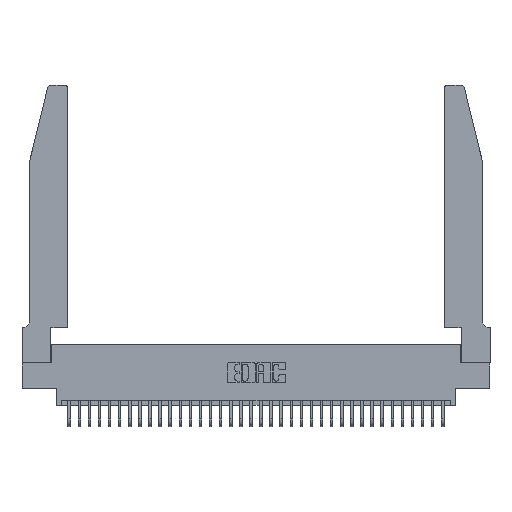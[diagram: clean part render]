
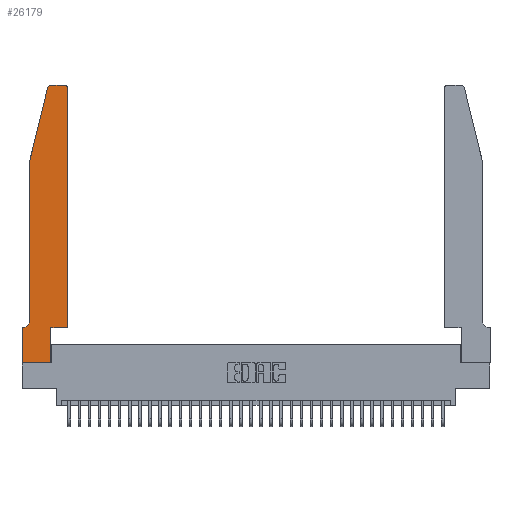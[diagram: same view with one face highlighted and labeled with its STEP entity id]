
A CAD part, top view. The second image highlights one B-rep face of the part: STEP entity #26179.
In plain terms, the highlighted planar face has unit normal (0, 0, 1).
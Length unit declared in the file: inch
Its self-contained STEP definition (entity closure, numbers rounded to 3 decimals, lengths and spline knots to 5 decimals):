
#414 = ORIENTED_EDGE ( 'NONE', *, *, #23794, .T. ) ;
#551 = EDGE_CURVE ( 'NONE', #29438, #9366, #21436, .T. ) ;
#573 = VERTEX_POINT ( 'NONE', #2773 ) ;
#674 = EDGE_CURVE ( 'NONE', #13265, #4782, #3933, .T. ) ;
#882 = CARTESIAN_POINT ( 'NONE',  ( 0.0055, 0.35, 0.37 ) ) ;
#1015 = DIRECTION ( 'NONE',  ( 0., 0., -1. ) ) ;
#1149 = AXIS2_PLACEMENT_3D ( 'NONE', #1820, #16306, #7664 ) ;
#1337 = VECTOR ( 'NONE', #31755, 39.37008 ) ;
#1820 = CARTESIAN_POINT ( 'NONE',  ( 0.284, 2.72, 0.37 ) ) ;
#2773 = CARTESIAN_POINT ( 'NONE',  ( 0.2865, 0., 0.37 ) ) ;
#2801 = CARTESIAN_POINT ( 'NONE',  ( 0.4205, 2.75, 0.37 ) ) ;
#2846 = ORIENTED_EDGE ( 'NONE', *, *, #32578, .T. ) ;
#3013 = EDGE_CURVE ( 'NONE', #4782, #20727, #36854, .T. ) ;
#3222 = ORIENTED_EDGE ( 'NONE', *, *, #8726, .T. ) ;
#3835 = DIRECTION ( 'NONE',  ( 1., 0., 0. ) ) ;
#3860 = ORIENTED_EDGE ( 'NONE', *, *, #13000, .T. ) ;
#3933 = LINE ( 'NONE', #31384, #4380 ) ;
#4380 = VECTOR ( 'NONE', #34259, 39.37008 ) ;
#4782 = VERTEX_POINT ( 'NONE', #15396 ) ;
#5200 = CARTESIAN_POINT ( 'NONE',  ( 0.2865, 0.35, 0.37 ) ) ;
#5363 = DIRECTION ( 'NONE',  ( 0., -1., 0. ) ) ;
#5480 = CARTESIAN_POINT ( 'NONE',  ( 0., 0., 0.37 ) ) ;
#5794 = CARTESIAN_POINT ( 'NONE',  ( 0.0755, 0.42, 0.37 ) ) ;
#5874 = CARTESIAN_POINT ( 'NONE',  ( 0.2605, 2.75, 0.37 ) ) ;
#6254 = EDGE_CURVE ( 'NONE', #573, #23156, #12474, .T. ) ;
#6316 = CARTESIAN_POINT ( 'NONE',  ( 0., 0., 0.37 ) ) ;
#6372 = CARTESIAN_POINT ( 'NONE',  ( 0.4505, 2.72, 0.37 ) ) ;
#6643 = CARTESIAN_POINT ( 'NONE',  ( 0.4505, 0.35, 0.37 ) ) ;
#6925 = CARTESIAN_POINT ( 'NONE',  ( 0., 0., 0.37 ) ) ;
#6975 = CARTESIAN_POINT ( 'NONE',  ( 0.0055, 0.42, 0.37 ) ) ;
#7664 = DIRECTION ( 'NONE',  ( 1., 0., 0. ) ) ;
#8200 = CIRCLE ( 'NONE', #1149, 0.03 ) ;
#8548 = CIRCLE ( 'NONE', #20520, 0.03 ) ;
#8627 = DIRECTION ( 'NONE',  ( 0., 1., 0. ) ) ;
#8636 = CARTESIAN_POINT ( 'NONE',  ( 0., 0.35, 0.37 ) ) ;
#8726 = EDGE_CURVE ( 'NONE', #18690, #29438, #17779, .T. ) ;
#9097 = DIRECTION ( 'NONE',  ( 0., 0., 1. ) ) ;
#9366 = VERTEX_POINT ( 'NONE', #5794 ) ;
#9663 = VECTOR ( 'NONE', #8627, 39.37008 ) ;
#10705 = LINE ( 'NONE', #5874, #1337 ) ;
#11784 = CARTESIAN_POINT ( 'NONE',  ( 0.25487, 2.72718, 0.37 ) ) ;
#12169 = ORIENTED_EDGE ( 'NONE', *, *, #28264, .T. ) ;
#12474 = LINE ( 'NONE', #5200, #14291 ) ;
#12577 = CARTESIAN_POINT ( 'NONE',  ( 0.0755, 2., 0.37 ) ) ;
#12782 = EDGE_CURVE ( 'NONE', #9366, #13265, #15246, .T. ) ;
#13000 = EDGE_CURVE ( 'NONE', #19731, #32443, #8548, .T. ) ;
#13149 = DIRECTION ( 'NONE',  ( 1., 0., 0. ) ) ;
#13265 = VERTEX_POINT ( 'NONE', #882 ) ;
#13441 = CARTESIAN_POINT ( 'NONE',  ( 0.0755, 2., 0.37 ) ) ;
#13556 = AXIS2_PLACEMENT_3D ( 'NONE', #6975, #1015, #24623 ) ;
#13829 = VECTOR ( 'NONE', #5363, 39.37008 ) ;
#13882 = LINE ( 'NONE', #6316, #31745 ) ;
#14057 = EDGE_CURVE ( 'NONE', #24492, #18690, #8200, .T. ) ;
#14215 = EDGE_LOOP ( 'NONE', ( #12169, #20579, #3222, #31974, #21783, #24744, #35398, #414, #27452, #2846, #31894, #3860 ) ) ;
#14291 = VECTOR ( 'NONE', #19339, 39.37008 ) ;
#14475 = VECTOR ( 'NONE', #34326, 39.37008 ) ;
#14519 = PLANE ( 'NONE',  #26498 ) ;
#14670 = LINE ( 'NONE', #26276, #9663 ) ;
#15246 = CIRCLE ( 'NONE', #13556, 0.07 ) ;
#15396 = CARTESIAN_POINT ( 'NONE',  ( 0., 0.35, 0.37 ) ) ;
#16199 = VERTEX_POINT ( 'NONE', #6643 ) ;
#16306 = DIRECTION ( 'NONE',  ( 0., 0., 1. ) ) ;
#17434 = CARTESIAN_POINT ( 'NONE',  ( 0.284, 2.75, 0.37 ) ) ;
#17779 = LINE ( 'NONE', #13441, #35224 ) ;
#18690 = VERTEX_POINT ( 'NONE', #11784 ) ;
#18780 = DIRECTION ( 'NONE',  ( 0., 0., 1. ) ) ;
#19339 = DIRECTION ( 'NONE',  ( 0., 1., 0. ) ) ;
#19497 = CARTESIAN_POINT ( 'NONE',  ( 0.0755, 2., 0.37 ) ) ;
#19563 = FACE_OUTER_BOUND ( 'NONE', #14215, .T. ) ;
#19731 = VERTEX_POINT ( 'NONE', #6372 ) ;
#20520 = AXIS2_PLACEMENT_3D ( 'NONE', #35878, #18780, #13149 ) ;
#20579 = ORIENTED_EDGE ( 'NONE', *, *, #14057, .T. ) ;
#20629 = CARTESIAN_POINT ( 'NONE',  ( 0.4505, 0.35, 0.37 ) ) ;
#20727 = VERTEX_POINT ( 'NONE', #6925 ) ;
#21436 = LINE ( 'NONE', #19497, #13829 ) ;
#21783 = ORIENTED_EDGE ( 'NONE', *, *, #12782, .T. ) ;
#23156 = VERTEX_POINT ( 'NONE', #28878 ) ;
#23794 = EDGE_CURVE ( 'NONE', #20727, #573, #13882, .T. ) ;
#24492 = VERTEX_POINT ( 'NONE', #17434 ) ;
#24623 = DIRECTION ( 'NONE',  ( -1., 0., 0. ) ) ;
#24744 = ORIENTED_EDGE ( 'NONE', *, *, #674, .T. ) ;
#24973 = DIRECTION ( 'NONE',  ( -0.239, -0.971, 0. ) ) ;
#25070 = EDGE_CURVE ( 'NONE', #16199, #19731, #14670, .T. ) ;
#26179 = ADVANCED_FACE ( 'NONE', ( #19563 ), #14519, .T. ) ;
#26276 = CARTESIAN_POINT ( 'NONE',  ( 0.4505, 0.35, 0.37 ) ) ;
#26498 = AXIS2_PLACEMENT_3D ( 'NONE', #8636, #9097, #29141 ) ;
#27452 = ORIENTED_EDGE ( 'NONE', *, *, #6254, .T. ) ;
#28264 = EDGE_CURVE ( 'NONE', #32443, #24492, #10705, .T. ) ;
#28878 = CARTESIAN_POINT ( 'NONE',  ( 0.2865, 0.35, 0.37 ) ) ;
#29097 = DIRECTION ( 'NONE',  ( 1., 0., 0. ) ) ;
#29141 = DIRECTION ( 'NONE',  ( 1., 0., 0. ) ) ;
#29438 = VERTEX_POINT ( 'NONE', #12577 ) ;
#31038 = VECTOR ( 'NONE', #3835, 39.37008 ) ;
#31384 = CARTESIAN_POINT ( 'NONE',  ( 0.0755, 0.35, 0.37 ) ) ;
#31745 = VECTOR ( 'NONE', #29097, 39.37008 ) ;
#31755 = DIRECTION ( 'NONE',  ( -1., 0., 0. ) ) ;
#31894 = ORIENTED_EDGE ( 'NONE', *, *, #25070, .T. ) ;
#31974 = ORIENTED_EDGE ( 'NONE', *, *, #551, .T. ) ;
#32443 = VERTEX_POINT ( 'NONE', #2801 ) ;
#32578 = EDGE_CURVE ( 'NONE', #23156, #16199, #32785, .T. ) ;
#32785 = LINE ( 'NONE', #20629, #31038 ) ;
#34259 = DIRECTION ( 'NONE',  ( -1., 0., 0. ) ) ;
#34326 = DIRECTION ( 'NONE',  ( 0., -1., 0. ) ) ;
#35224 = VECTOR ( 'NONE', #24973, 39.37008 ) ;
#35398 = ORIENTED_EDGE ( 'NONE', *, *, #3013, .T. ) ;
#35878 = CARTESIAN_POINT ( 'NONE',  ( 0.4205, 2.72, 0.37 ) ) ;
#36854 = LINE ( 'NONE', #5480, #14475 ) ;
